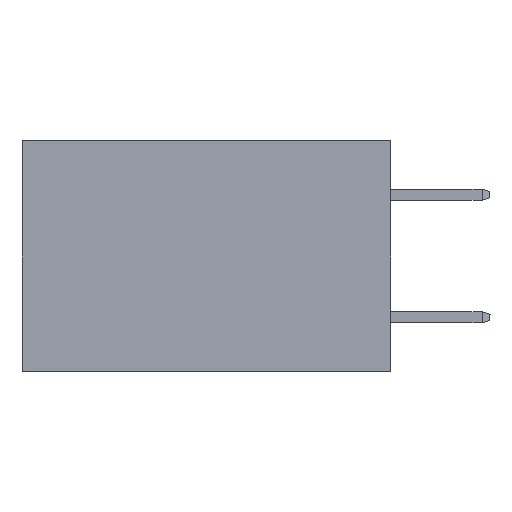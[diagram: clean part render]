
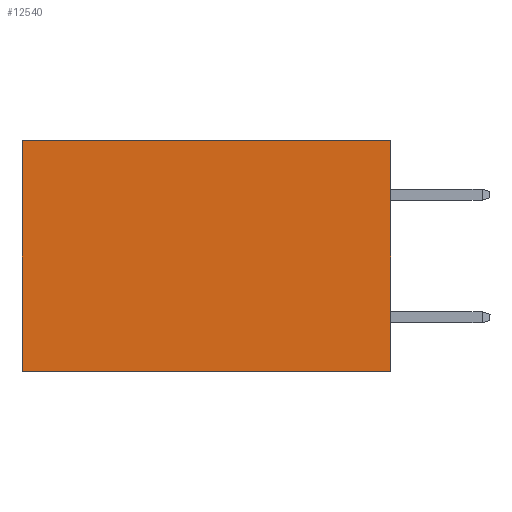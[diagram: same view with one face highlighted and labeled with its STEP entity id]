
A CAD part, left-side view. The second image highlights one B-rep face of the part: STEP entity #12540.
In plain terms, the highlighted planar face has unit normal (-1, 0, 0).
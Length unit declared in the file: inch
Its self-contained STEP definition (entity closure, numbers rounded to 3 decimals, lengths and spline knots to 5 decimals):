
#53 = VECTOR ( 'NONE', #673, 39.37008 ) ;
#112 = EDGE_CURVE ( 'NONE', #12211, #12029, #13624, .T. ) ;
#673 = DIRECTION ( 'NONE',  ( 0., 0., -1. ) ) ;
#764 = CARTESIAN_POINT ( 'NONE',  ( 0.2875, 0.6, -0.375 ) ) ;
#2346 = FACE_OUTER_BOUND ( 'NONE', #5130, .T. ) ;
#2955 = DIRECTION ( 'NONE',  ( 0., 0., -1. ) ) ;
#3129 = LINE ( 'NONE', #5209, #6494 ) ;
#3291 = CARTESIAN_POINT ( 'NONE',  ( 0.2875, 0.6, 0. ) ) ;
#3380 = ORIENTED_EDGE ( 'NONE', *, *, #12240, .T. ) ;
#3614 = ORIENTED_EDGE ( 'NONE', *, *, #4144, .F. ) ;
#3680 = ORIENTED_EDGE ( 'NONE', *, *, #112, .F. ) ;
#4144 = EDGE_CURVE ( 'NONE', #6362, #12211, #15009, .T. ) ;
#4978 = EDGE_CURVE ( 'NONE', #11830, #12029, #9198, .T. ) ;
#5130 = EDGE_LOOP ( 'NONE', ( #13679, #3680, #3614, #3380 ) ) ;
#5209 = CARTESIAN_POINT ( 'NONE',  ( 0.2875, 0., 0. ) ) ;
#5370 = CARTESIAN_POINT ( 'NONE',  ( 0.2875, 0., -0.375 ) ) ;
#5773 = VECTOR ( 'NONE', #10697, 39.37008 ) ;
#6362 = VERTEX_POINT ( 'NONE', #13894 ) ;
#6494 = VECTOR ( 'NONE', #11195, 39.37008 ) ;
#7464 = CARTESIAN_POINT ( 'NONE',  ( 0.2875, 0.6, -0.375 ) ) ;
#7705 = CARTESIAN_POINT ( 'NONE',  ( 0.2875, 0., -0.375 ) ) ;
#8235 = DIRECTION ( 'NONE',  ( 0., 0., -1. ) ) ;
#8262 = CARTESIAN_POINT ( 'NONE',  ( 0.2875, 0., -0.375 ) ) ;
#8330 = DIRECTION ( 'NONE',  ( 1., 0., 0. ) ) ;
#9198 = LINE ( 'NONE', #764, #53 ) ;
#10512 = PLANE ( 'NONE',  #14667 ) ;
#10697 = DIRECTION ( 'NONE',  ( 0., 1., 0. ) ) ;
#11195 = DIRECTION ( 'NONE',  ( 0., 1., 0. ) ) ;
#11236 = VECTOR ( 'NONE', #2955, 39.37008 ) ;
#11722 = CARTESIAN_POINT ( 'NONE',  ( 0.2875, 0., -0.375 ) ) ;
#11830 = VERTEX_POINT ( 'NONE', #3291 ) ;
#12029 = VERTEX_POINT ( 'NONE', #7464 ) ;
#12211 = VERTEX_POINT ( 'NONE', #5370 ) ;
#12240 = EDGE_CURVE ( 'NONE', #6362, #11830, #3129, .T. ) ;
#12540 = ADVANCED_FACE ( 'NONE', ( #2346 ), #10512, .F. ) ;
#13624 = LINE ( 'NONE', #8262, #5773 ) ;
#13679 = ORIENTED_EDGE ( 'NONE', *, *, #4978, .T. ) ;
#13894 = CARTESIAN_POINT ( 'NONE',  ( 0.2875, 0., 0. ) ) ;
#14667 = AXIS2_PLACEMENT_3D ( 'NONE', #11722, #8330, #8235 ) ;
#15009 = LINE ( 'NONE', #7705, #11236 ) ;
